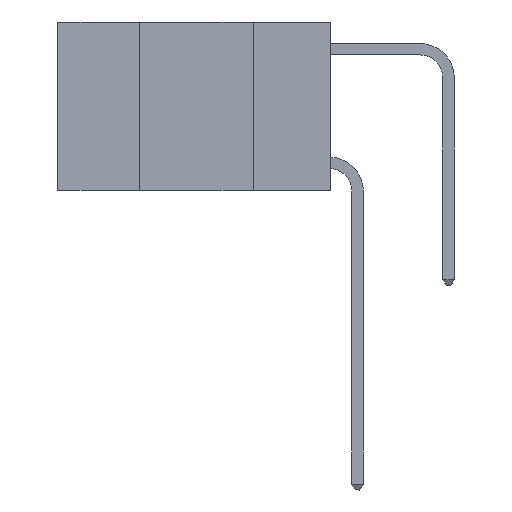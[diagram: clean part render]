
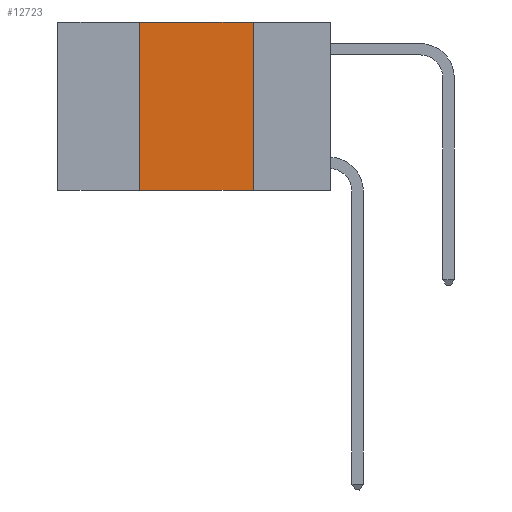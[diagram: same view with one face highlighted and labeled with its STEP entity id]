
A CAD part, left-side view. The second image highlights one B-rep face of the part: STEP entity #12723.
In plain terms, the highlighted planar face has unit normal (-1, 0, 0).
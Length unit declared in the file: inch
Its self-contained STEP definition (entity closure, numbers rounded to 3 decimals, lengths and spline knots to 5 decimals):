
#1133 = CARTESIAN_POINT ( 'NONE',  ( 0., 0.17, -0.37 ) ) ;
#1143 = ORIENTED_EDGE ( 'NONE', *, *, #16446, .F. ) ;
#1307 = ORIENTED_EDGE ( 'NONE', *, *, #4897, .T. ) ;
#2195 = CARTESIAN_POINT ( 'NONE',  ( 0., 0.17, 0. ) ) ;
#2896 = EDGE_CURVE ( 'NONE', #4949, #7942, #15060, .T. ) ;
#3152 = CARTESIAN_POINT ( 'NONE',  ( 0., 0.6, 0. ) ) ;
#3293 = AXIS2_PLACEMENT_3D ( 'NONE', #10305, #4158, #14826 ) ;
#4106 = VECTOR ( 'NONE', #19250, 39.37008 ) ;
#4158 = DIRECTION ( 'NONE',  ( 1., 0., 0. ) ) ;
#4239 = ORIENTED_EDGE ( 'NONE', *, *, #2896, .F. ) ;
#4897 = EDGE_CURVE ( 'NONE', #4949, #16756, #13141, .T. ) ;
#4949 = VERTEX_POINT ( 'NONE', #19147 ) ;
#5209 = DIRECTION ( 'NONE',  ( 0., -1., 0. ) ) ;
#5253 = CARTESIAN_POINT ( 'NONE',  ( 0., 0.17, 0. ) ) ;
#6581 = CARTESIAN_POINT ( 'NONE',  ( 0., 0.6, -0.37 ) ) ;
#6833 = CARTESIAN_POINT ( 'NONE',  ( 0., 0.42, 0. ) ) ;
#6902 = LINE ( 'NONE', #3152, #12178 ) ;
#7467 = CARTESIAN_POINT ( 'NONE',  ( 0., 0.42, 0. ) ) ;
#7942 = VERTEX_POINT ( 'NONE', #7467 ) ;
#10305 = CARTESIAN_POINT ( 'NONE',  ( 0., 0.6, 0. ) ) ;
#11416 = DIRECTION ( 'NONE',  ( 0., 0., -1. ) ) ;
#11448 = ORIENTED_EDGE ( 'NONE', *, *, #12291, .F. ) ;
#12178 = VECTOR ( 'NONE', #18359, 39.37008 ) ;
#12291 = EDGE_CURVE ( 'NONE', #15211, #16756, #16101, .T. ) ;
#12297 = VECTOR ( 'NONE', #11416, 39.37008 ) ;
#12723 = ADVANCED_FACE ( 'NONE', ( #18189 ), #14882, .F. ) ;
#13141 = LINE ( 'NONE', #6581, #17387 ) ;
#13182 = EDGE_LOOP ( 'NONE', ( #11448, #1143, #4239, #1307 ) ) ;
#14826 = DIRECTION ( 'NONE',  ( 0., 0., -1. ) ) ;
#14882 = PLANE ( 'NONE',  #3293 ) ;
#15060 = LINE ( 'NONE', #6833, #4106 ) ;
#15211 = VERTEX_POINT ( 'NONE', #2195 ) ;
#16101 = LINE ( 'NONE', #5253, #12297 ) ;
#16446 = EDGE_CURVE ( 'NONE', #7942, #15211, #6902, .T. ) ;
#16756 = VERTEX_POINT ( 'NONE', #1133 ) ;
#17387 = VECTOR ( 'NONE', #5209, 39.37008 ) ;
#18189 = FACE_OUTER_BOUND ( 'NONE', #13182, .T. ) ;
#18359 = DIRECTION ( 'NONE',  ( 0., -1., 0. ) ) ;
#19147 = CARTESIAN_POINT ( 'NONE',  ( 0., 0.42, -0.37 ) ) ;
#19250 = DIRECTION ( 'NONE',  ( 0., 0., 1. ) ) ;
